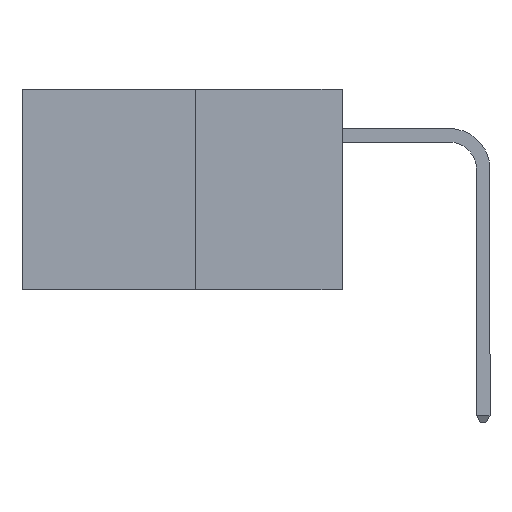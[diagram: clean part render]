
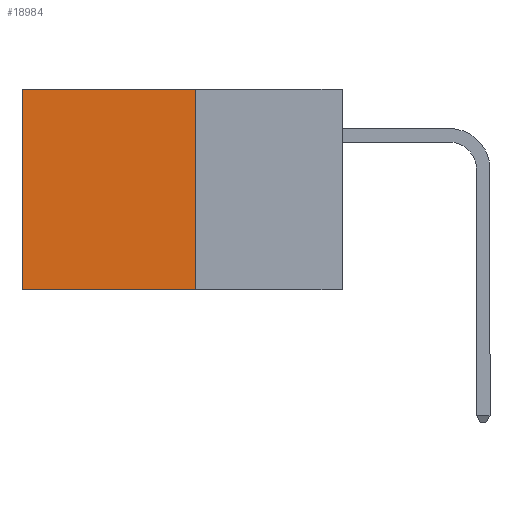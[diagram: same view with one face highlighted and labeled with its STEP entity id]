
A CAD part, left-side view. The second image highlights one B-rep face of the part: STEP entity #18984.
In plain terms, the highlighted planar face has unit normal (-1, 0, 0).
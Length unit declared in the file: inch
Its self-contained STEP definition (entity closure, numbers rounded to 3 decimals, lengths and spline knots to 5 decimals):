
#80 = VERTEX_POINT ( 'NONE', #10444 ) ;
#2438 = EDGE_CURVE ( 'NONE', #8976, #80, #7801, .T. ) ;
#3503 = DIRECTION ( 'NONE',  ( 0., 1., 0. ) ) ;
#4076 = CARTESIAN_POINT ( 'NONE',  ( 0.277, 0.59, -0.37 ) ) ;
#4193 = CARTESIAN_POINT ( 'NONE',  ( 0.277, 0.27, 0. ) ) ;
#5361 = EDGE_CURVE ( 'NONE', #8976, #18603, #22585, .T. ) ;
#5432 = ORIENTED_EDGE ( 'NONE', *, *, #11871, .T. ) ;
#5863 = CARTESIAN_POINT ( 'NONE',  ( 0.277, 0.27, -0.37 ) ) ;
#7532 = AXIS2_PLACEMENT_3D ( 'NONE', #10136, #25601, #12317 ) ;
#7624 = DIRECTION ( 'NONE',  ( 0., 0., -1. ) ) ;
#7801 = LINE ( 'NONE', #9942, #18162 ) ;
#8976 = VERTEX_POINT ( 'NONE', #4193 ) ;
#9033 = VECTOR ( 'NONE', #7624, 39.37008 ) ;
#9565 = FACE_OUTER_BOUND ( 'NONE', #16777, .T. ) ;
#9724 = LINE ( 'NONE', #9830, #9033 ) ;
#9830 = CARTESIAN_POINT ( 'NONE',  ( 0.277, 0.59, -0.37 ) ) ;
#9942 = CARTESIAN_POINT ( 'NONE',  ( 0.277, 0.27, -0.37 ) ) ;
#10136 = CARTESIAN_POINT ( 'NONE',  ( 0.277, 0.27, -0.37 ) ) ;
#10169 = EDGE_CURVE ( 'NONE', #80, #17888, #16411, .T. ) ;
#10301 = DIRECTION ( 'NONE',  ( 0., 1., 0. ) ) ;
#10444 = CARTESIAN_POINT ( 'NONE',  ( 0.277, 0.27, -0.37 ) ) ;
#11482 = ORIENTED_EDGE ( 'NONE', *, *, #10169, .F. ) ;
#11871 = EDGE_CURVE ( 'NONE', #18603, #17888, #9724, .T. ) ;
#12317 = DIRECTION ( 'NONE',  ( 0., 0., -1. ) ) ;
#15590 = ORIENTED_EDGE ( 'NONE', *, *, #5361, .T. ) ;
#16411 = LINE ( 'NONE', #5863, #23703 ) ;
#16777 = EDGE_LOOP ( 'NONE', ( #5432, #11482, #19940, #15590 ) ) ;
#17888 = VERTEX_POINT ( 'NONE', #4076 ) ;
#18162 = VECTOR ( 'NONE', #18755, 39.37008 ) ;
#18603 = VERTEX_POINT ( 'NONE', #24376 ) ;
#18755 = DIRECTION ( 'NONE',  ( 0., 0., -1. ) ) ;
#18982 = CARTESIAN_POINT ( 'NONE',  ( 0.277, 0.27, 0. ) ) ;
#18984 = ADVANCED_FACE ( 'NONE', ( #9565 ), #23410, .F. ) ;
#19940 = ORIENTED_EDGE ( 'NONE', *, *, #2438, .F. ) ;
#22585 = LINE ( 'NONE', #18982, #28482 ) ;
#23410 = PLANE ( 'NONE',  #7532 ) ;
#23703 = VECTOR ( 'NONE', #10301, 39.37008 ) ;
#24376 = CARTESIAN_POINT ( 'NONE',  ( 0.277, 0.59, 0. ) ) ;
#25601 = DIRECTION ( 'NONE',  ( 1., 0., 0. ) ) ;
#28482 = VECTOR ( 'NONE', #3503, 39.37008 ) ;
